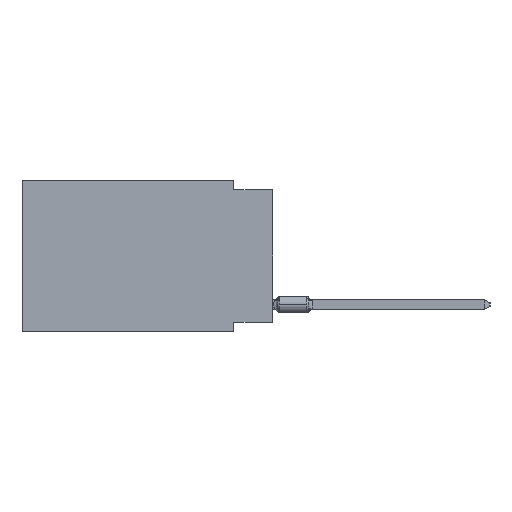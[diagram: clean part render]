
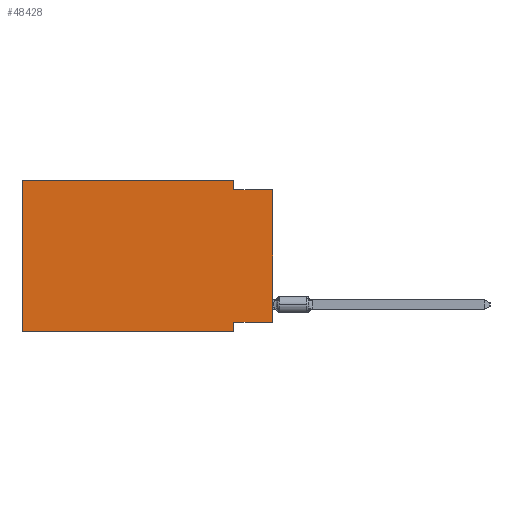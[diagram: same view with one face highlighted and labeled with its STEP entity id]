
A CAD part, left-side view. The second image highlights one B-rep face of the part: STEP entity #48428.
In plain terms, the highlighted planar face has unit normal (-1, 0, 0).
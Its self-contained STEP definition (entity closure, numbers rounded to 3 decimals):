
#84 = ORIENTED_EDGE ( 'NONE', *, *, #25024, .F. ) ;
#389 = VERTEX_POINT ( 'NONE', #72655 ) ;
#1838 = PLANE ( 'NONE',  #11719 ) ;
#4533 = VECTOR ( 'NONE', #16518, 1000. ) ;
#8151 = DIRECTION ( 'NONE',  ( 0., 0., 1. ) ) ;
#9759 = DIRECTION ( 'NONE',  ( 0., 0., -1. ) ) ;
#10310 = ORIENTED_EDGE ( 'NONE', *, *, #19410, .F. ) ;
#10800 = LINE ( 'NONE', #61469, #19996 ) ;
#11229 = EDGE_CURVE ( 'NONE', #389, #62265, #76088, .T. ) ;
#11719 = AXIS2_PLACEMENT_3D ( 'NONE', #37599, #73708, #43150 ) ;
#11872 = CARTESIAN_POINT ( 'NONE',  ( 0., 2.54, -9.906 ) ) ;
#13269 = ORIENTED_EDGE ( 'NONE', *, *, #42460, .T. ) ;
#15708 = CARTESIAN_POINT ( 'NONE',  ( 0., 2.54, 0. ) ) ;
#16518 = DIRECTION ( 'NONE',  ( 0., -1., 0. ) ) ;
#17005 = CARTESIAN_POINT ( 'NONE',  ( 0., 2.54, -9.906 ) ) ;
#18725 = CARTESIAN_POINT ( 'NONE',  ( 0., 0., -9.271 ) ) ;
#19267 = CARTESIAN_POINT ( 'NONE',  ( 0., 16.383, 0. ) ) ;
#19369 = DIRECTION ( 'NONE',  ( 0., 0., 1. ) ) ;
#19410 = EDGE_CURVE ( 'NONE', #33776, #52724, #73909, .T. ) ;
#19996 = VECTOR ( 'NONE', #19369, 1000. ) ;
#20295 = CARTESIAN_POINT ( 'NONE',  ( 0., 0., -0.635 ) ) ;
#23679 = EDGE_LOOP ( 'NONE', ( #13269, #27671, #56946, #42121, #47992, #51110, #84, #10310 ) ) ;
#25024 = EDGE_CURVE ( 'NONE', #52724, #62265, #48809, .T. ) ;
#25080 = DIRECTION ( 'NONE',  ( 0., -1., 0. ) ) ;
#26803 = VECTOR ( 'NONE', #9759, 1000. ) ;
#27671 = ORIENTED_EDGE ( 'NONE', *, *, #39157, .F. ) ;
#28229 = VECTOR ( 'NONE', #8151, 1000. ) ;
#31054 = LINE ( 'NONE', #20295, #64138 ) ;
#31748 = VECTOR ( 'NONE', #56815, 1000. ) ;
#32772 = EDGE_CURVE ( 'NONE', #68467, #50049, #70095, .T. ) ;
#33763 = VERTEX_POINT ( 'NONE', #63000 ) ;
#33776 = VERTEX_POINT ( 'NONE', #57820 ) ;
#34390 = CARTESIAN_POINT ( 'NONE',  ( 0., 16.383, -9.906 ) ) ;
#36108 = DIRECTION ( 'NONE',  ( 0., 0., -1. ) ) ;
#36373 = CARTESIAN_POINT ( 'NONE',  ( 0., 2.54, 0. ) ) ;
#37599 = CARTESIAN_POINT ( 'NONE',  ( 0., 16.383, 0. ) ) ;
#39157 = EDGE_CURVE ( 'NONE', #50049, #33763, #31054, .T. ) ;
#42121 = ORIENTED_EDGE ( 'NONE', *, *, #66968, .F. ) ;
#42460 = EDGE_CURVE ( 'NONE', #33776, #33763, #10800, .T. ) ;
#43150 = DIRECTION ( 'NONE',  ( 0., 0., -1. ) ) ;
#43285 = CARTESIAN_POINT ( 'NONE',  ( 0., 2.54, -0.635 ) ) ;
#44289 = LINE ( 'NONE', #19267, #28229 ) ;
#47992 = ORIENTED_EDGE ( 'NONE', *, *, #74277, .F. ) ;
#48428 = ADVANCED_FACE ( 'NONE', ( #67363 ), #1838, .F. ) ;
#48809 = LINE ( 'NONE', #11872, #74275 ) ;
#50049 = VERTEX_POINT ( 'NONE', #43285 ) ;
#51110 = ORIENTED_EDGE ( 'NONE', *, *, #11229, .T. ) ;
#51654 = LINE ( 'NONE', #69500, #31748 ) ;
#52724 = VERTEX_POINT ( 'NONE', #54462 ) ;
#53401 = VECTOR ( 'NONE', #55662, 1000. ) ;
#54462 = CARTESIAN_POINT ( 'NONE',  ( 0., 2.54, -9.271 ) ) ;
#55662 = DIRECTION ( 'NONE',  ( 0., 1., 0. ) ) ;
#56815 = DIRECTION ( 'NONE',  ( 0., -1., 0. ) ) ;
#56946 = ORIENTED_EDGE ( 'NONE', *, *, #32772, .F. ) ;
#57820 = CARTESIAN_POINT ( 'NONE',  ( 0., 0., -9.271 ) ) ;
#61469 = CARTESIAN_POINT ( 'NONE',  ( 0., 0., 0. ) ) ;
#62265 = VERTEX_POINT ( 'NONE', #17005 ) ;
#63000 = CARTESIAN_POINT ( 'NONE',  ( 0., 0., -0.635 ) ) ;
#64088 = VERTEX_POINT ( 'NONE', #69278 ) ;
#64138 = VECTOR ( 'NONE', #25080, 1000. ) ;
#66968 = EDGE_CURVE ( 'NONE', #64088, #68467, #51654, .T. ) ;
#67363 = FACE_OUTER_BOUND ( 'NONE', #23679, .T. ) ;
#68467 = VERTEX_POINT ( 'NONE', #36373 ) ;
#69278 = CARTESIAN_POINT ( 'NONE',  ( 0., 16.383, 0. ) ) ;
#69500 = CARTESIAN_POINT ( 'NONE',  ( 0., 16.383, 0. ) ) ;
#70095 = LINE ( 'NONE', #15708, #26803 ) ;
#72655 = CARTESIAN_POINT ( 'NONE',  ( 0., 16.383, -9.906 ) ) ;
#73708 = DIRECTION ( 'NONE',  ( 1., 0., 0. ) ) ;
#73909 = LINE ( 'NONE', #18725, #53401 ) ;
#74275 = VECTOR ( 'NONE', #36108, 1000. ) ;
#74277 = EDGE_CURVE ( 'NONE', #389, #64088, #44289, .T. ) ;
#76088 = LINE ( 'NONE', #34390, #4533 ) ;
